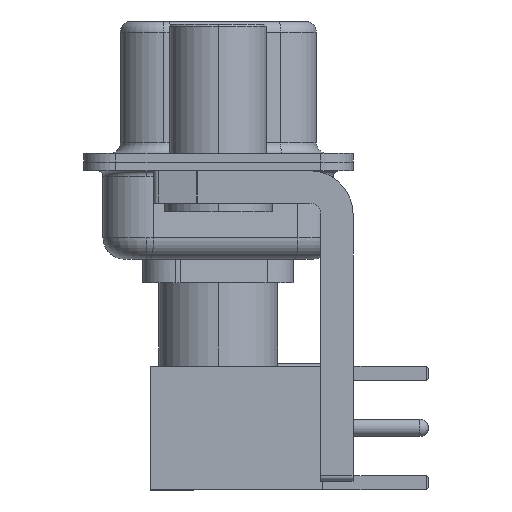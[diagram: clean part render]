
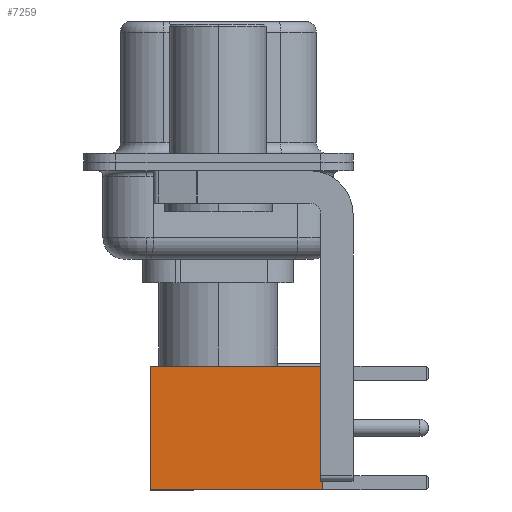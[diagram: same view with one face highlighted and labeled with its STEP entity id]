
A CAD part, left-side view. The second image highlights one B-rep face of the part: STEP entity #7259.
In plain terms, the highlighted face is planar.
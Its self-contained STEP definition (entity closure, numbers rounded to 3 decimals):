
#57 = CARTESIAN_POINT ( 'NONE',  ( 0., 2.875, 0. ) ) ;
#210 = VERTEX_POINT ( 'NONE', #8731 ) ;
#314 = VECTOR ( 'NONE', #23609, 1000. ) ;
#3310 = CARTESIAN_POINT ( 'NONE',  ( 2.875, 2.875, 0. ) ) ;
#4298 = VECTOR ( 'NONE', #9614, 1000. ) ;
#4765 = CARTESIAN_POINT ( 'NONE',  ( 0., 2.875, 8. ) ) ;
#4777 = ORIENTED_EDGE ( 'NONE', *, *, #8100, .T. ) ;
#4917 = LINE ( 'NONE', #4765, #4298 ) ;
#5070 = EDGE_LOOP ( 'NONE', ( #4777, #26298, #18908, #29743 ) ) ;
#6011 = CARTESIAN_POINT ( 'NONE',  ( -2.875, 2.875, 0. ) ) ;
#7259 = ADVANCED_FACE ( 'NONE', ( #26578 ), #24709, .T. ) ;
#7309 = LINE ( 'NONE', #57, #9637 ) ;
#8004 = DIRECTION ( 'NONE',  ( 0., 1., 0. ) ) ;
#8100 = EDGE_CURVE ( 'NONE', #210, #17042, #19227, .T. ) ;
#8731 = CARTESIAN_POINT ( 'NONE',  ( 2.875, 2.875, 8. ) ) ;
#9614 = DIRECTION ( 'NONE',  ( -1., 0., 0. ) ) ;
#9637 = VECTOR ( 'NONE', #27690, 1000. ) ;
#9721 = CARTESIAN_POINT ( 'NONE',  ( 2.875, 2.875, 0. ) ) ;
#10318 = CARTESIAN_POINT ( 'NONE',  ( -2.875, 2.875, 8. ) ) ;
#10408 = CARTESIAN_POINT ( 'NONE',  ( 2.875, 2.875, 0. ) ) ;
#13424 = CARTESIAN_POINT ( 'NONE',  ( -2.875, 2.875, 0. ) ) ;
#15998 = DIRECTION ( 'NONE',  ( 0., 0., -1. ) ) ;
#17042 = VERTEX_POINT ( 'NONE', #10408 ) ;
#17637 = VECTOR ( 'NONE', #15998, 1000. ) ;
#18110 = EDGE_CURVE ( 'NONE', #20663, #28172, #22937, .T. ) ;
#18908 = ORIENTED_EDGE ( 'NONE', *, *, #18110, .F. ) ;
#19227 = LINE ( 'NONE', #9721, #314 ) ;
#19575 = AXIS2_PLACEMENT_3D ( 'NONE', #3310, #8004, #26426 ) ;
#20663 = VERTEX_POINT ( 'NONE', #10318 ) ;
#21422 = EDGE_CURVE ( 'NONE', #210, #20663, #4917, .T. ) ;
#22012 = EDGE_CURVE ( 'NONE', #17042, #28172, #7309, .T. ) ;
#22937 = LINE ( 'NONE', #13424, #17637 ) ;
#23609 = DIRECTION ( 'NONE',  ( 0., 0., -1. ) ) ;
#24709 = PLANE ( 'NONE',  #19575 ) ;
#26298 = ORIENTED_EDGE ( 'NONE', *, *, #22012, .T. ) ;
#26426 = DIRECTION ( 'NONE',  ( 0., 0., 1. ) ) ;
#26578 = FACE_OUTER_BOUND ( 'NONE', #5070, .T. ) ;
#27690 = DIRECTION ( 'NONE',  ( -1., 0., 0. ) ) ;
#28172 = VERTEX_POINT ( 'NONE', #6011 ) ;
#29743 = ORIENTED_EDGE ( 'NONE', *, *, #21422, .F. ) ;
